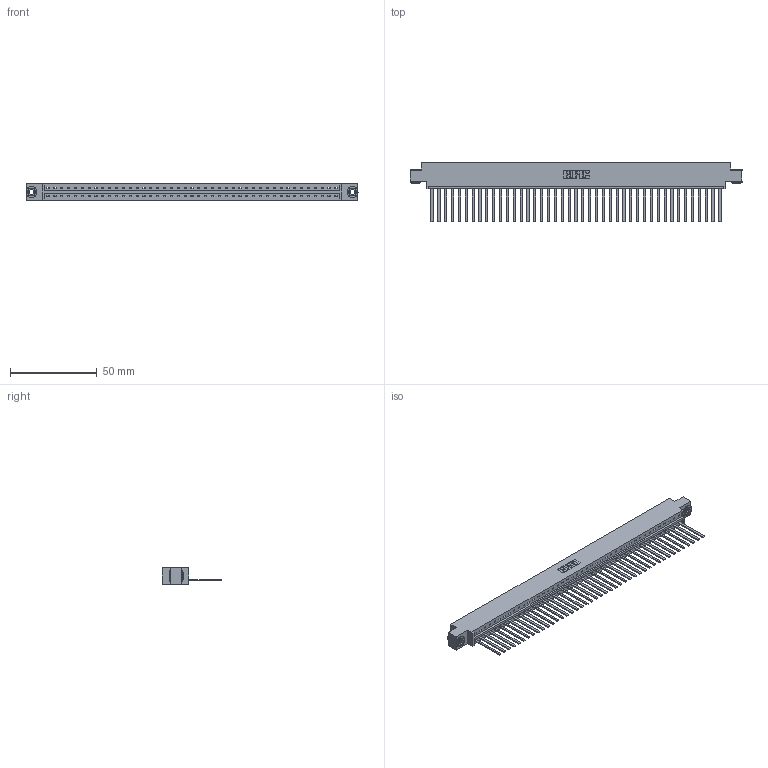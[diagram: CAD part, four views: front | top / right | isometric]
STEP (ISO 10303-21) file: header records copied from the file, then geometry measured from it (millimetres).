
FILE_DESCRIPTION (( 'STEP AP203' ), '1' );
FILE_NAME ('333-043-544-603.STEP', '2018-08-03T20:35:58', ( '' ), ( '' ), 'SwSTEP 2.0', 'SolidWorks 2016', '' );
FILE_SCHEMA (( 'CONFIG_CONTROL_DESIGN' ));
Length unit declared in the file: inch
Products named in the file (4): 345-292-001_345-293-144; 345-250-002_345-250-002-102; 333-043-544-603; 333 Part_Offset - .156 Dia - TH
Assembly tree (46 placements, depth 2):
  333-043-544-603
    333 Part_Offset - .156 Dia - TH
    345-292-001_345-293-144  x43
    345-250-002_345-250-002-102  x2
Bounding box: 191.92 x 34.3 x 9.4 mm (x, y, z)
Volume: 19611 mm3; surface area: 23270.2 mm2
Topology: 46 solids, 46 shells, 2392 faces, 7193 edges, 4734 vertices
Faces by surface type: plane 1718, cylinder 666, cone 8
Entity records: 26756 total; most frequent: CARTESIAN_POINT 4594, ORIENTED_EDGE 4566, DIRECTION 3903, EDGE_CURVE 2283, VECTOR 2135, LINE 2135, VERTEX_POINT 1518, AXIS2_PLACEMENT_3D 884
